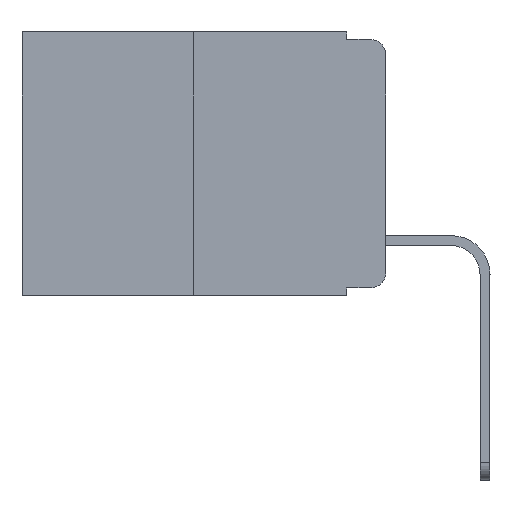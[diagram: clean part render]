
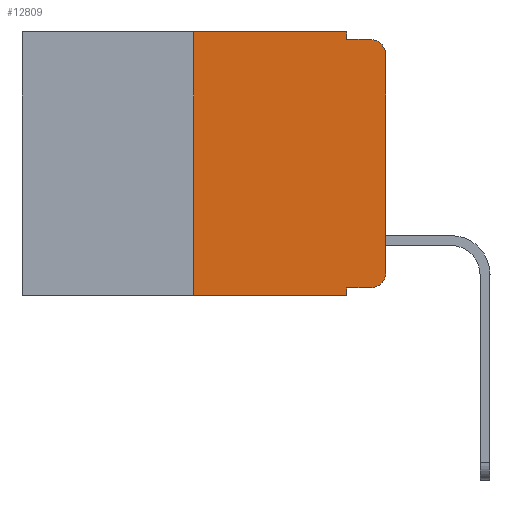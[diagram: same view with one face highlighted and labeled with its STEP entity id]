
A CAD part, left-side view. The second image highlights one B-rep face of the part: STEP entity #12809.
In plain terms, the highlighted planar face has unit normal (-1, 0, 0).
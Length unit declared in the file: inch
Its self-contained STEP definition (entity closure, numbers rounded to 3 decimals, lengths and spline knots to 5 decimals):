
#82 = EDGE_LOOP ( 'NONE', ( #11216, #22325, #720, #5254, #4881, #1314, #4096, #18570, #8470, #10064 ) ) ;
#321 = AXIS2_PLACEMENT_3D ( 'NONE', #10835, #16647, #5053 ) ;
#396 = CARTESIAN_POINT ( 'NONE',  ( 0., 0.02, -0.313 ) ) ;
#503 = EDGE_CURVE ( 'NONE', #24423, #12686, #14673, .T. ) ;
#720 = ORIENTED_EDGE ( 'NONE', *, *, #2323, .F. ) ;
#724 = CARTESIAN_POINT ( 'NONE',  ( 0., 0.051, -0.333 ) ) ;
#1314 = ORIENTED_EDGE ( 'NONE', *, *, #23586, .F. ) ;
#1628 = EDGE_CURVE ( 'NONE', #8314, #8323, #15815, .T. ) ;
#2179 = EDGE_CURVE ( 'NONE', #19939, #8314, #3081, .T. ) ;
#2257 = AXIS2_PLACEMENT_3D ( 'NONE', #5493, #7504, #7421 ) ;
#2323 = EDGE_CURVE ( 'NONE', #10702, #8323, #11583, .T. ) ;
#2387 = CIRCLE ( 'NONE', #21665, 0.02 ) ;
#3081 = LINE ( 'NONE', #12795, #24582 ) ;
#3172 = PLANE ( 'NONE',  #321 ) ;
#3910 = CARTESIAN_POINT ( 'NONE',  ( 0., 0.25, 0. ) ) ;
#4096 = ORIENTED_EDGE ( 'NONE', *, *, #11582, .T. ) ;
#4311 = EDGE_CURVE ( 'NONE', #23302, #18106, #14846, .T. ) ;
#4881 = ORIENTED_EDGE ( 'NONE', *, *, #503, .F. ) ;
#5053 = DIRECTION ( 'NONE',  ( 0., 0., -1. ) ) ;
#5254 = ORIENTED_EDGE ( 'NONE', *, *, #8435, .F. ) ;
#5480 = DIRECTION ( 'NONE',  ( 0., 0., 1. ) ) ;
#5493 = CARTESIAN_POINT ( 'NONE',  ( 0., 0.02, -0.03 ) ) ;
#6440 = DIRECTION ( 'NONE',  ( 0., -1., 0. ) ) ;
#6780 = FACE_OUTER_BOUND ( 'NONE', #82, .T. ) ;
#7061 = DIRECTION ( 'NONE',  ( 0., 0., -1. ) ) ;
#7314 = VECTOR ( 'NONE', #20684, 39.37008 ) ;
#7421 = DIRECTION ( 'NONE',  ( 0., 0., -1. ) ) ;
#7504 = DIRECTION ( 'NONE',  ( -1., 0., 0. ) ) ;
#8059 = LINE ( 'NONE', #15686, #9286 ) ;
#8310 = LINE ( 'NONE', #22795, #14712 ) ;
#8314 = VERTEX_POINT ( 'NONE', #17379 ) ;
#8323 = VERTEX_POINT ( 'NONE', #9726 ) ;
#8435 = EDGE_CURVE ( 'NONE', #12686, #10702, #16971, .T. ) ;
#8470 = ORIENTED_EDGE ( 'NONE', *, *, #4311, .T. ) ;
#8484 = VECTOR ( 'NONE', #6440, 39.37008 ) ;
#8880 = EDGE_CURVE ( 'NONE', #18106, #19939, #2387, .T. ) ;
#8963 = LINE ( 'NONE', #18620, #23171 ) ;
#9286 = VECTOR ( 'NONE', #19439, 39.37008 ) ;
#9715 = VERTEX_POINT ( 'NONE', #17057 ) ;
#9726 = CARTESIAN_POINT ( 'NONE',  ( 0., 0.02, -0.01 ) ) ;
#10064 = ORIENTED_EDGE ( 'NONE', *, *, #8880, .T. ) ;
#10268 = DIRECTION ( 'NONE',  ( -1., 0., 0. ) ) ;
#10528 = DIRECTION ( 'NONE',  ( 0., 0., 1. ) ) ;
#10702 = VERTEX_POINT ( 'NONE', #11181 ) ;
#10835 = CARTESIAN_POINT ( 'NONE',  ( 0., 0.473, 0. ) ) ;
#11181 = CARTESIAN_POINT ( 'NONE',  ( 0., 0.051, -0.01 ) ) ;
#11216 = ORIENTED_EDGE ( 'NONE', *, *, #2179, .T. ) ;
#11242 = VECTOR ( 'NONE', #14165, 39.37008 ) ;
#11284 = EDGE_CURVE ( 'NONE', #23302, #19178, #8963, .T. ) ;
#11534 = DIRECTION ( 'NONE',  ( 0., -1., 0. ) ) ;
#11582 = EDGE_CURVE ( 'NONE', #9715, #19178, #8059, .T. ) ;
#11583 = LINE ( 'NONE', #13209, #7314 ) ;
#12390 = CARTESIAN_POINT ( 'NONE',  ( 0., 0.051, -0.343 ) ) ;
#12556 = VECTOR ( 'NONE', #11534, 39.37008 ) ;
#12686 = VERTEX_POINT ( 'NONE', #17970 ) ;
#12795 = CARTESIAN_POINT ( 'NONE',  ( 0., 0., 0. ) ) ;
#12809 = ADVANCED_FACE ( 'NONE', ( #6780 ), #3172, .F. ) ;
#13209 = CARTESIAN_POINT ( 'NONE',  ( 0., 0.051, -0.01 ) ) ;
#14165 = DIRECTION ( 'NONE',  ( 0., 0., -1. ) ) ;
#14673 = LINE ( 'NONE', #23086, #12556 ) ;
#14712 = VECTOR ( 'NONE', #5480, 39.37008 ) ;
#14813 = CARTESIAN_POINT ( 'NONE',  ( 0., 0.02, -0.333 ) ) ;
#14846 = LINE ( 'NONE', #18000, #8484 ) ;
#15686 = CARTESIAN_POINT ( 'NONE',  ( 0., 0.473, -0.343 ) ) ;
#15815 = CIRCLE ( 'NONE', #2257, 0.02 ) ;
#16647 = DIRECTION ( 'NONE',  ( 1., 0., 0. ) ) ;
#16971 = LINE ( 'NONE', #23771, #11242 ) ;
#17057 = CARTESIAN_POINT ( 'NONE',  ( 0., 0.25, -0.343 ) ) ;
#17379 = CARTESIAN_POINT ( 'NONE',  ( 0., 0., -0.03 ) ) ;
#17970 = CARTESIAN_POINT ( 'NONE',  ( 0., 0.051, 0. ) ) ;
#18000 = CARTESIAN_POINT ( 'NONE',  ( 0., 0.051, -0.333 ) ) ;
#18106 = VERTEX_POINT ( 'NONE', #14813 ) ;
#18570 = ORIENTED_EDGE ( 'NONE', *, *, #11284, .F. ) ;
#18620 = CARTESIAN_POINT ( 'NONE',  ( 0., 0.051, 0. ) ) ;
#19178 = VERTEX_POINT ( 'NONE', #12390 ) ;
#19439 = DIRECTION ( 'NONE',  ( 0., -1., 0. ) ) ;
#19939 = VERTEX_POINT ( 'NONE', #19991 ) ;
#19991 = CARTESIAN_POINT ( 'NONE',  ( 0., 0., -0.313 ) ) ;
#20684 = DIRECTION ( 'NONE',  ( 0., -1., 0. ) ) ;
#21665 = AXIS2_PLACEMENT_3D ( 'NONE', #396, #10268, #21711 ) ;
#21711 = DIRECTION ( 'NONE',  ( 0., 0., -1. ) ) ;
#22325 = ORIENTED_EDGE ( 'NONE', *, *, #1628, .T. ) ;
#22795 = CARTESIAN_POINT ( 'NONE',  ( 0., 0.25, 0. ) ) ;
#23086 = CARTESIAN_POINT ( 'NONE',  ( 0., 0.473, 0. ) ) ;
#23171 = VECTOR ( 'NONE', #7061, 39.37008 ) ;
#23302 = VERTEX_POINT ( 'NONE', #724 ) ;
#23586 = EDGE_CURVE ( 'NONE', #9715, #24423, #8310, .T. ) ;
#23771 = CARTESIAN_POINT ( 'NONE',  ( 0., 0.051, 0. ) ) ;
#24423 = VERTEX_POINT ( 'NONE', #3910 ) ;
#24582 = VECTOR ( 'NONE', #10528, 39.37008 ) ;
